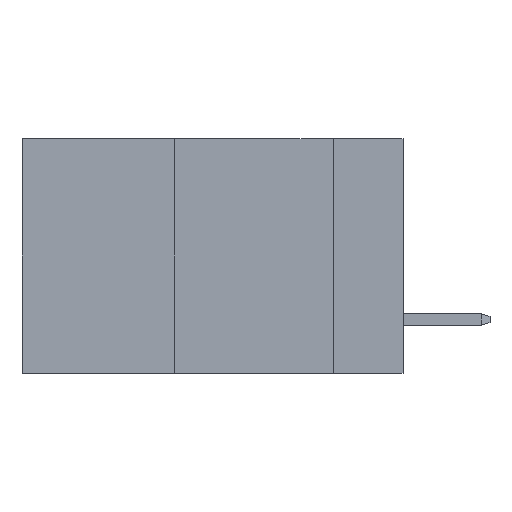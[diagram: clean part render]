
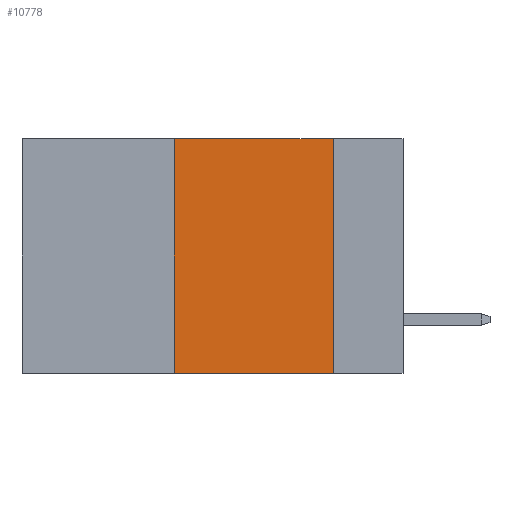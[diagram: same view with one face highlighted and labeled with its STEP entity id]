
A CAD part, left-side view. The second image highlights one B-rep face of the part: STEP entity #10778.
In plain terms, the highlighted planar face has unit normal (-1, 0, 0).
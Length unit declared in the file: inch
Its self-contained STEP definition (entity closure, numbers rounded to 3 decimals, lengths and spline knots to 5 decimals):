
#111 = CARTESIAN_POINT ( 'NONE',  ( 0., 0.36, 0. ) ) ;
#1907 = VECTOR ( 'NONE', #13607, 39.37008 ) ;
#1918 = CARTESIAN_POINT ( 'NONE',  ( 0., 0.36, 0. ) ) ;
#1926 = ORIENTED_EDGE ( 'NONE', *, *, #10928, .F. ) ;
#2864 = CARTESIAN_POINT ( 'NONE',  ( 0., 0.6, 0. ) ) ;
#3443 = LINE ( 'NONE', #13282, #1907 ) ;
#3570 = VECTOR ( 'NONE', #5268, 39.37008 ) ;
#3661 = EDGE_LOOP ( 'NONE', ( #7956, #1926, #5961, #12878 ) ) ;
#3971 = DIRECTION ( 'NONE',  ( 0., 0., 1. ) ) ;
#5020 = CARTESIAN_POINT ( 'NONE',  ( 0., 0.6, 0. ) ) ;
#5268 = DIRECTION ( 'NONE',  ( 0., -1., 0. ) ) ;
#5961 = ORIENTED_EDGE ( 'NONE', *, *, #8761, .F. ) ;
#6030 = FACE_OUTER_BOUND ( 'NONE', #3661, .T. ) ;
#6414 = EDGE_CURVE ( 'NONE', #8138, #12693, #8706, .T. ) ;
#7367 = CARTESIAN_POINT ( 'NONE',  ( 0., 0.11, 0. ) ) ;
#7956 = ORIENTED_EDGE ( 'NONE', *, *, #13123, .F. ) ;
#8138 = VERTEX_POINT ( 'NONE', #13190 ) ;
#8706 = LINE ( 'NONE', #9790, #13754 ) ;
#8761 = EDGE_CURVE ( 'NONE', #8138, #15178, #15544, .T. ) ;
#8852 = AXIS2_PLACEMENT_3D ( 'NONE', #5020, #16027, #15011 ) ;
#9790 = CARTESIAN_POINT ( 'NONE',  ( 0., 0.6, -0.37 ) ) ;
#9887 = VECTOR ( 'NONE', #3971, 39.37008 ) ;
#10001 = PLANE ( 'NONE',  #8852 ) ;
#10778 = ADVANCED_FACE ( 'NONE', ( #6030 ), #10001, .F. ) ;
#10928 = EDGE_CURVE ( 'NONE', #15178, #15800, #11735, .T. ) ;
#11735 = LINE ( 'NONE', #2864, #3570 ) ;
#12593 = DIRECTION ( 'NONE',  ( 0., -1., 0. ) ) ;
#12693 = VERTEX_POINT ( 'NONE', #15860 ) ;
#12878 = ORIENTED_EDGE ( 'NONE', *, *, #6414, .T. ) ;
#13123 = EDGE_CURVE ( 'NONE', #15800, #12693, #3443, .T. ) ;
#13190 = CARTESIAN_POINT ( 'NONE',  ( 0., 0.36, -0.37 ) ) ;
#13282 = CARTESIAN_POINT ( 'NONE',  ( 0., 0.11, 0. ) ) ;
#13607 = DIRECTION ( 'NONE',  ( 0., 0., -1. ) ) ;
#13754 = VECTOR ( 'NONE', #12593, 39.37008 ) ;
#15011 = DIRECTION ( 'NONE',  ( 0., 0., -1. ) ) ;
#15178 = VERTEX_POINT ( 'NONE', #1918 ) ;
#15544 = LINE ( 'NONE', #111, #9887 ) ;
#15800 = VERTEX_POINT ( 'NONE', #7367 ) ;
#15860 = CARTESIAN_POINT ( 'NONE',  ( 0., 0.11, -0.37 ) ) ;
#16027 = DIRECTION ( 'NONE',  ( 1., 0., 0. ) ) ;
